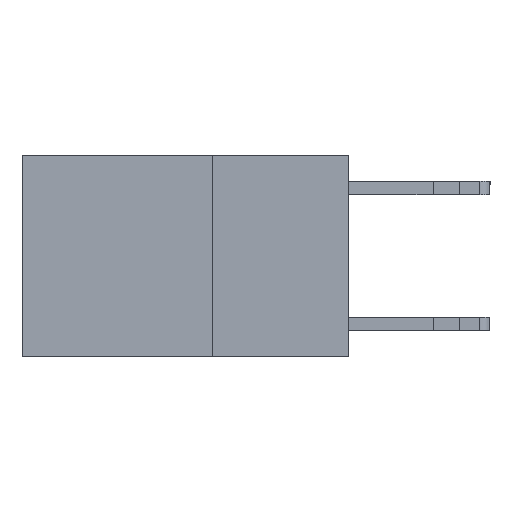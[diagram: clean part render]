
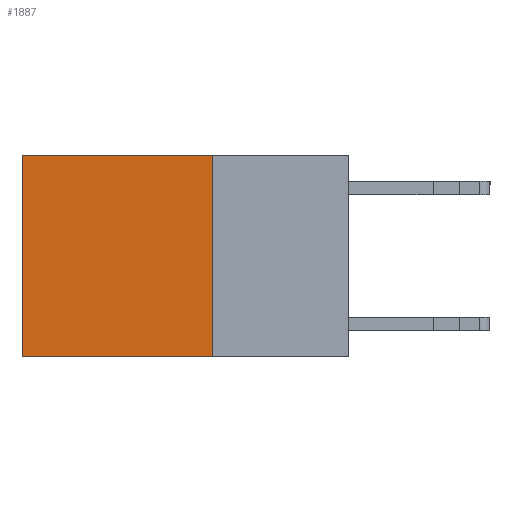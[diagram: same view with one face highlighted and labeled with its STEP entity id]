
A CAD part, left-side view. The second image highlights one B-rep face of the part: STEP entity #1887.
In plain terms, the highlighted planar face has unit normal (-1, 0, 0).
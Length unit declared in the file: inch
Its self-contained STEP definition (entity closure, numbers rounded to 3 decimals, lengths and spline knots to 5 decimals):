
#6 = PLANE ( 'NONE',  #7363 ) ;
#93 = DIRECTION ( 'NONE',  ( 0., 0., -1. ) ) ;
#682 = CARTESIAN_POINT ( 'NONE',  ( 0.2625, 0.25, -0.37 ) ) ;
#1299 = ORIENTED_EDGE ( 'NONE', *, *, #7987, .T. ) ;
#1468 = VECTOR ( 'NONE', #16033, 39.37008 ) ;
#1754 = EDGE_CURVE ( 'NONE', #8070, #8824, #4701, .T. ) ;
#1887 = ADVANCED_FACE ( 'NONE', ( #3941 ), #6, .F. ) ;
#1959 = ORIENTED_EDGE ( 'NONE', *, *, #1754, .F. ) ;
#2306 = CARTESIAN_POINT ( 'NONE',  ( 0.2625, 0.25, 0. ) ) ;
#2974 = CARTESIAN_POINT ( 'NONE',  ( 0.2625, 0.25, 0. ) ) ;
#3781 = CARTESIAN_POINT ( 'NONE',  ( 0.2625, 0.25, 0. ) ) ;
#3941 = FACE_OUTER_BOUND ( 'NONE', #8682, .T. ) ;
#4400 = DIRECTION ( 'NONE',  ( 0., 1., 0. ) ) ;
#4701 = LINE ( 'NONE', #6110, #5509 ) ;
#4800 = CARTESIAN_POINT ( 'NONE',  ( 0.2625, 0.6, 0. ) ) ;
#4806 = CARTESIAN_POINT ( 'NONE',  ( 0.2625, 0.6, -0.37 ) ) ;
#4867 = DIRECTION ( 'NONE',  ( 0., 0., -1. ) ) ;
#5509 = VECTOR ( 'NONE', #4867, 39.37008 ) ;
#5652 = LINE ( 'NONE', #2974, #12589 ) ;
#6110 = CARTESIAN_POINT ( 'NONE',  ( 0.2625, 0.25, 0. ) ) ;
#7363 = AXIS2_PLACEMENT_3D ( 'NONE', #3781, #11536, #93 ) ;
#7987 = EDGE_CURVE ( 'NONE', #8070, #16010, #5652, .T. ) ;
#8070 = VERTEX_POINT ( 'NONE', #2306 ) ;
#8682 = EDGE_LOOP ( 'NONE', ( #10527, #13058, #1959, #1299 ) ) ;
#8824 = VERTEX_POINT ( 'NONE', #14932 ) ;
#9861 = DIRECTION ( 'NONE',  ( 0., 0., -1. ) ) ;
#10080 = CARTESIAN_POINT ( 'NONE',  ( 0.2625, 0.6, 0. ) ) ;
#10527 = ORIENTED_EDGE ( 'NONE', *, *, #11069, .T. ) ;
#11069 = EDGE_CURVE ( 'NONE', #16010, #13802, #16062, .T. ) ;
#11536 = DIRECTION ( 'NONE',  ( 1., 0., 0. ) ) ;
#12589 = VECTOR ( 'NONE', #4400, 39.37008 ) ;
#13058 = ORIENTED_EDGE ( 'NONE', *, *, #15913, .F. ) ;
#13802 = VERTEX_POINT ( 'NONE', #4806 ) ;
#14871 = LINE ( 'NONE', #682, #1468 ) ;
#14932 = CARTESIAN_POINT ( 'NONE',  ( 0.2625, 0.25, -0.37 ) ) ;
#15913 = EDGE_CURVE ( 'NONE', #8824, #13802, #14871, .T. ) ;
#16010 = VERTEX_POINT ( 'NONE', #10080 ) ;
#16014 = VECTOR ( 'NONE', #9861, 39.37008 ) ;
#16033 = DIRECTION ( 'NONE',  ( 0., 1., 0. ) ) ;
#16062 = LINE ( 'NONE', #4800, #16014 ) ;
